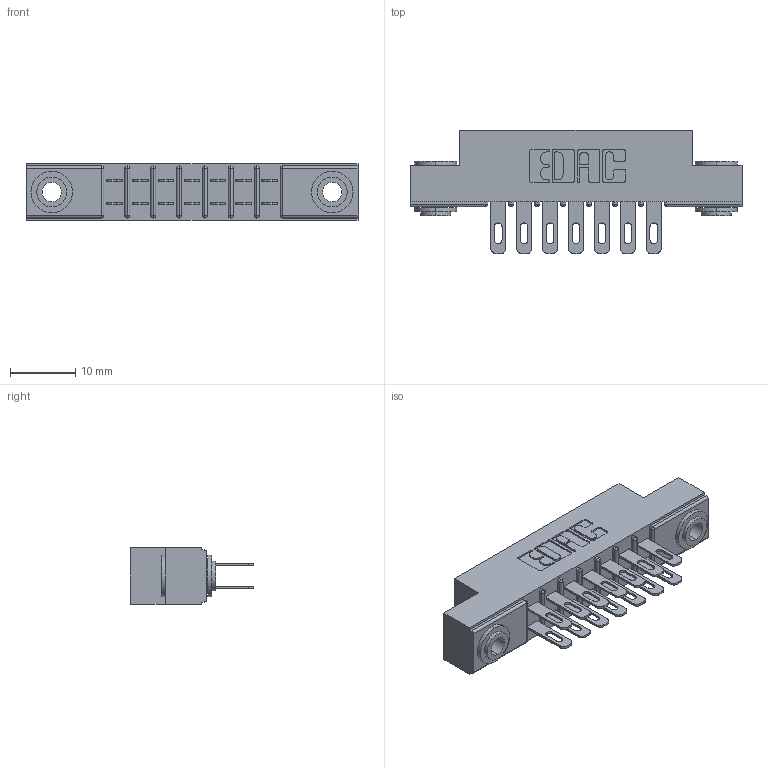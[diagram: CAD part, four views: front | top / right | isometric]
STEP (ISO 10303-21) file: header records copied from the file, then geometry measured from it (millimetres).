
FILE_DESCRIPTION (( 'STEP AP203' ), '1' );
FILE_NAME ('305-014-500-203.STEP', '2019-09-09T11:35:02', ( '' ), ( '' ), 'SwSTEP 2.0', 'SolidWorks 2016', '' );
FILE_SCHEMA (( 'CONFIG_CONTROL_DESIGN' ));
Length unit declared in the file: inch
Products named in the file (4): 305-290-001_500; 305-014-500-203; 345-250-002_345-250-002-102; 305 Part_.156 Dia
Assembly tree (17 placements, depth 2):
  305-014-500-203
    305 Part_.156 Dia
    305-290-001_500  x14
    345-250-002_345-250-002-102  x2
Bounding box: 50.75 x 18.85 x 8.71 mm (x, y, z)
Volume: 3246.2 mm3; surface area: 5753.1 mm2
Topology: 17 solids, 17 shells, 868 faces, 2437 edges, 1582 vertices
Faces by surface type: plane 484, cylinder 348, sphere 28, cone 8
Entity records: 12927 total; most frequent: CARTESIAN_POINT 2120, DIRECTION 2097, ORIENTED_EDGE 2090, EDGE_CURVE 1045, VECTOR 795, LINE 795, VERTEX_POINT 674, AXIS2_PLACEMENT_3D 651
